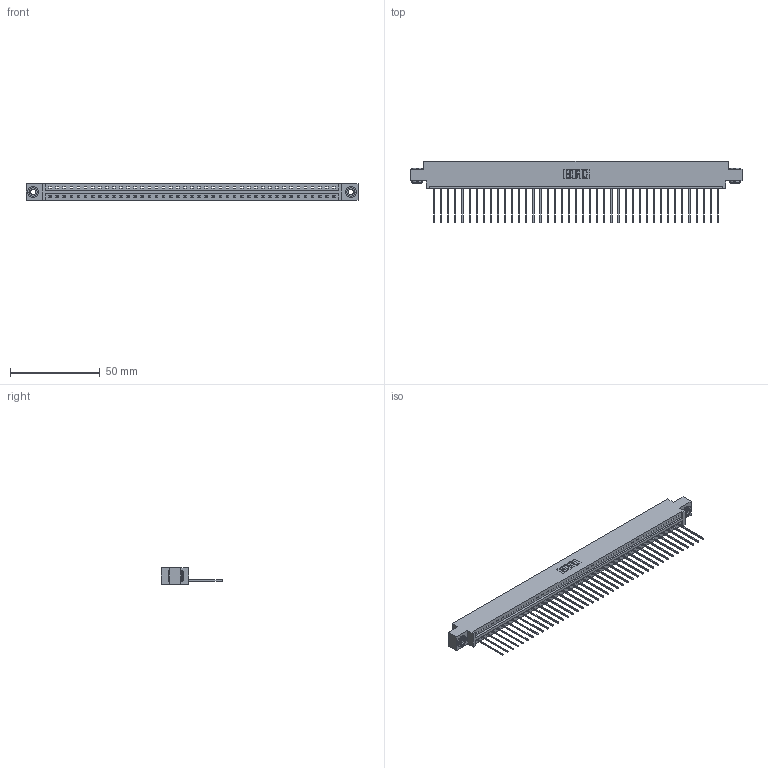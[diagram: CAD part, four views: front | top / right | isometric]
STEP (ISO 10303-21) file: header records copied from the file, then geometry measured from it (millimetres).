
FILE_DESCRIPTION (( 'STEP AP203' ), '1' );
FILE_NAME ('337-041-541-603.STEP', '2019-10-01T21:01:14', ( '' ), ( '' ), 'SwSTEP 2.0', 'SolidWorks 2016', '' );
FILE_SCHEMA (( 'CONFIG_CONTROL_DESIGN' ));
Length unit declared in the file: inch
Products named in the file (4): 337-041-541-603; 337 Part_0.170 Offset - 0.156 Dia-TH; 345-250-002_345-250-002-102; 345-292-001_345-293-141
Assembly tree (44 placements, depth 2):
  337-041-541-603
    337 Part_0.170 Offset - 0.156 Dia-TH
    345-292-001_345-293-141  x41
    345-250-002_345-250-002-102  x2
Bounding box: 185.47 x 34.3 x 9.4 mm (x, y, z)
Volume: 19301.3 mm3; surface area: 21100.8 mm2
Topology: 44 solids, 44 shells, 2698 faces, 8107 edges, 5346 vertices
Faces by surface type: plane 1970, cylinder 720, cone 8
Entity records: 31406 total; most frequent: CARTESIAN_POINT 5448, ORIENTED_EDGE 5418, DIRECTION 4621, EDGE_CURVE 2709, LINE 2557, VECTOR 2557, VERTEX_POINT 1802, AXIS2_PLACEMENT_3D 1032
